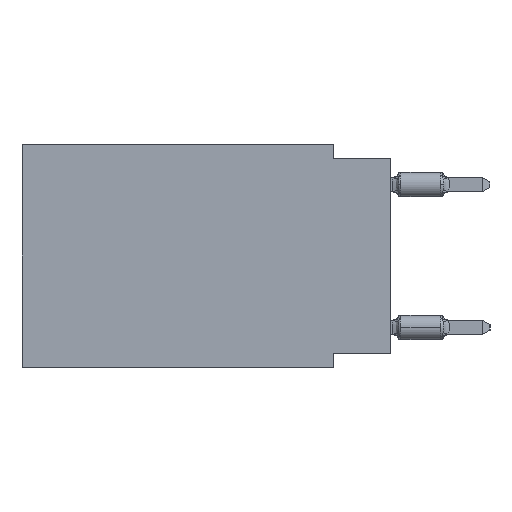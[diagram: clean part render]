
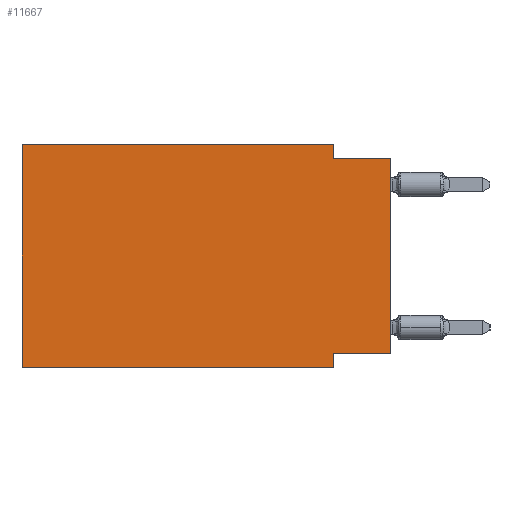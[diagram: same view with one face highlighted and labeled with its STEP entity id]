
A CAD part, left-side view. The second image highlights one B-rep face of the part: STEP entity #11667.
In plain terms, the highlighted planar face has unit normal (-1, 0, 0).
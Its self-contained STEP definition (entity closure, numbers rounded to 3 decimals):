
#897 = CARTESIAN_POINT ( 'NONE',  ( 0., 2.54, -9.906 ) ) ;
#1280 = LINE ( 'NONE', #7054, #16477 ) ;
#1319 = LINE ( 'NONE', #15437, #34120 ) ;
#1338 = EDGE_CURVE ( 'NONE', #9466, #32531, #6924, .T. ) ;
#1742 = CARTESIAN_POINT ( 'NONE',  ( 0., 2.54, 0. ) ) ;
#3714 = CARTESIAN_POINT ( 'NONE',  ( 0., 0., 0. ) ) ;
#4486 = VERTEX_POINT ( 'NONE', #12218 ) ;
#4675 = DIRECTION ( 'NONE',  ( 0., -1., 0. ) ) ;
#4786 = VECTOR ( 'NONE', #26918, 1000. ) ;
#5995 = VERTEX_POINT ( 'NONE', #23937 ) ;
#6924 = LINE ( 'NONE', #21405, #36154 ) ;
#7054 = CARTESIAN_POINT ( 'NONE',  ( 0., 16.383, -9.906 ) ) ;
#7452 = LINE ( 'NONE', #22431, #18360 ) ;
#8361 = CARTESIAN_POINT ( 'NONE',  ( 0., 16.383, 0. ) ) ;
#8818 = FACE_OUTER_BOUND ( 'NONE', #29946, .T. ) ;
#9466 = VERTEX_POINT ( 'NONE', #8361 ) ;
#10460 = ORIENTED_EDGE ( 'NONE', *, *, #13118, .T. ) ;
#11056 = CARTESIAN_POINT ( 'NONE',  ( 0., 2.54, 0. ) ) ;
#11355 = ORIENTED_EDGE ( 'NONE', *, *, #21685, .F. ) ;
#11667 = ADVANCED_FACE ( 'NONE', ( #8818 ), #19770, .F. ) ;
#11702 = DIRECTION ( 'NONE',  ( 0., -1., 0. ) ) ;
#12218 = CARTESIAN_POINT ( 'NONE',  ( 0., 2.54, -9.271 ) ) ;
#12640 = DIRECTION ( 'NONE',  ( 0., 0., 1. ) ) ;
#13118 = EDGE_CURVE ( 'NONE', #5995, #33865, #34950, .T. ) ;
#13134 = CARTESIAN_POINT ( 'NONE',  ( 0., 0., -9.271 ) ) ;
#13651 = ORIENTED_EDGE ( 'NONE', *, *, #35251, .F. ) ;
#14384 = EDGE_CURVE ( 'NONE', #15118, #35131, #1280, .T. ) ;
#15111 = ORIENTED_EDGE ( 'NONE', *, *, #14384, .T. ) ;
#15118 = VERTEX_POINT ( 'NONE', #25751 ) ;
#15437 = CARTESIAN_POINT ( 'NONE',  ( 0., 16.383, 0. ) ) ;
#16238 = ORIENTED_EDGE ( 'NONE', *, *, #35889, .F. ) ;
#16477 = VECTOR ( 'NONE', #18557, 1000. ) ;
#17059 = ORIENTED_EDGE ( 'NONE', *, *, #28065, .F. ) ;
#17340 = DIRECTION ( 'NONE',  ( 0., 0., -1. ) ) ;
#18360 = VECTOR ( 'NONE', #36766, 1000. ) ;
#18557 = DIRECTION ( 'NONE',  ( 0., -1., 0. ) ) ;
#19428 = ORIENTED_EDGE ( 'NONE', *, *, #29002, .F. ) ;
#19770 = PLANE ( 'NONE',  #27355 ) ;
#20677 = CARTESIAN_POINT ( 'NONE',  ( 0., 0., -0.635 ) ) ;
#20751 = CARTESIAN_POINT ( 'NONE',  ( 0., 0., -0.635 ) ) ;
#21405 = CARTESIAN_POINT ( 'NONE',  ( 0., 16.383, 0. ) ) ;
#21685 = EDGE_CURVE ( 'NONE', #24543, #33865, #34026, .T. ) ;
#22168 = VECTOR ( 'NONE', #11702, 1000. ) ;
#22231 = LINE ( 'NONE', #13134, #30143 ) ;
#22431 = CARTESIAN_POINT ( 'NONE',  ( 0., 2.54, -9.906 ) ) ;
#23937 = CARTESIAN_POINT ( 'NONE',  ( 0., 0., -9.271 ) ) ;
#24543 = VERTEX_POINT ( 'NONE', #31558 ) ;
#24959 = ORIENTED_EDGE ( 'NONE', *, *, #1338, .F. ) ;
#25034 = DIRECTION ( 'NONE',  ( 0., 1., 0. ) ) ;
#25751 = CARTESIAN_POINT ( 'NONE',  ( 0., 16.383, -9.906 ) ) ;
#26918 = DIRECTION ( 'NONE',  ( 0., 0., 1. ) ) ;
#27355 = AXIS2_PLACEMENT_3D ( 'NONE', #34097, #28129, #17340 ) ;
#27965 = LINE ( 'NONE', #11056, #29891 ) ;
#28065 = EDGE_CURVE ( 'NONE', #5995, #4486, #22231, .T. ) ;
#28129 = DIRECTION ( 'NONE',  ( 1., 0., 0. ) ) ;
#29002 = EDGE_CURVE ( 'NONE', #4486, #35131, #7452, .T. ) ;
#29891 = VECTOR ( 'NONE', #33740, 1000. ) ;
#29946 = EDGE_LOOP ( 'NONE', ( #10460, #11355, #13651, #24959, #16238, #15111, #19428, #17059 ) ) ;
#30143 = VECTOR ( 'NONE', #25034, 1000. ) ;
#31558 = CARTESIAN_POINT ( 'NONE',  ( 0., 2.54, -0.635 ) ) ;
#32531 = VERTEX_POINT ( 'NONE', #1742 ) ;
#33740 = DIRECTION ( 'NONE',  ( 0., 0., -1. ) ) ;
#33865 = VERTEX_POINT ( 'NONE', #20751 ) ;
#34026 = LINE ( 'NONE', #20677, #22168 ) ;
#34097 = CARTESIAN_POINT ( 'NONE',  ( 0., 16.383, 0. ) ) ;
#34120 = VECTOR ( 'NONE', #12640, 1000. ) ;
#34950 = LINE ( 'NONE', #3714, #4786 ) ;
#35131 = VERTEX_POINT ( 'NONE', #897 ) ;
#35251 = EDGE_CURVE ( 'NONE', #32531, #24543, #27965, .T. ) ;
#35889 = EDGE_CURVE ( 'NONE', #15118, #9466, #1319, .T. ) ;
#36154 = VECTOR ( 'NONE', #4675, 1000. ) ;
#36766 = DIRECTION ( 'NONE',  ( 0., 0., -1. ) ) ;
